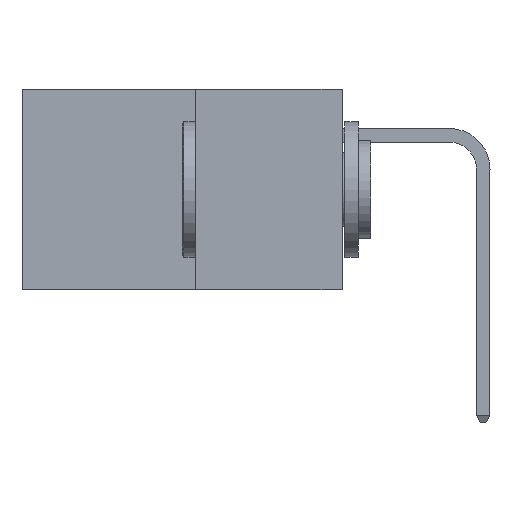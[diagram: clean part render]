
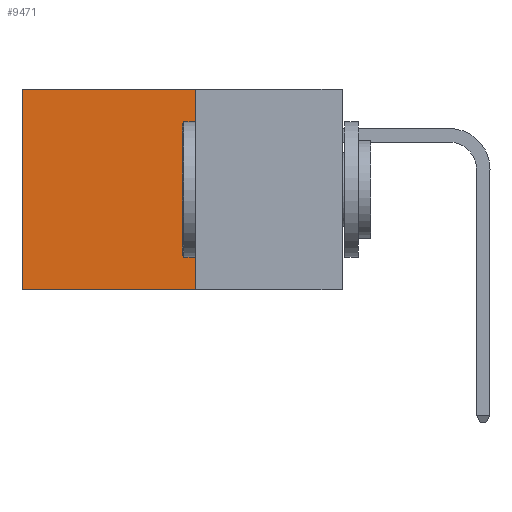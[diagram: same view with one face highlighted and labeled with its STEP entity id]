
A CAD part, left-side view. The second image highlights one B-rep face of the part: STEP entity #9471.
In plain terms, the highlighted planar face has unit normal (-1, 0, 0).
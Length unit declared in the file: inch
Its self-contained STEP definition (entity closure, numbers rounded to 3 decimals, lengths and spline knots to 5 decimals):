
#259 = VECTOR ( 'NONE', #9777, 39.37008 ) ;
#512 = CARTESIAN_POINT ( 'NONE',  ( 0.277, 0.59, -0.37 ) ) ;
#874 = PLANE ( 'NONE',  #8660 ) ;
#1087 = EDGE_CURVE ( 'NONE', #30436, #26529, #21596, .T. ) ;
#2315 = CARTESIAN_POINT ( 'NONE',  ( 0.277, 0.27, 0. ) ) ;
#2369 = CARTESIAN_POINT ( 'NONE',  ( 0.277, 0.27, -0.37 ) ) ;
#3928 = CARTESIAN_POINT ( 'NONE',  ( 0.277, 0.27, -0.37 ) ) ;
#5010 = ORIENTED_EDGE ( 'NONE', *, *, #18793, .F. ) ;
#5689 = VECTOR ( 'NONE', #22698, 39.37008 ) ;
#6069 = DIRECTION ( 'NONE',  ( 0., 0., -1. ) ) ;
#7139 = LINE ( 'NONE', #12357, #259 ) ;
#7997 = VECTOR ( 'NONE', #11887, 39.37008 ) ;
#8660 = AXIS2_PLACEMENT_3D ( 'NONE', #18874, #21423, #6069 ) ;
#9471 = ADVANCED_FACE ( 'NONE', ( #9560 ), #874, .F. ) ;
#9560 = FACE_OUTER_BOUND ( 'NONE', #23953, .T. ) ;
#9777 = DIRECTION ( 'NONE',  ( 0., 0., -1. ) ) ;
#9941 = ORIENTED_EDGE ( 'NONE', *, *, #1087, .F. ) ;
#11887 = DIRECTION ( 'NONE',  ( 0., 0., -1. ) ) ;
#12357 = CARTESIAN_POINT ( 'NONE',  ( 0.277, 0.59, -0.37 ) ) ;
#14771 = CARTESIAN_POINT ( 'NONE',  ( 0.277, 0.27, 0. ) ) ;
#18793 = EDGE_CURVE ( 'NONE', #26529, #22008, #29172, .T. ) ;
#18874 = CARTESIAN_POINT ( 'NONE',  ( 0.277, 0.27, -0.37 ) ) ;
#19292 = DIRECTION ( 'NONE',  ( 0., 1., 0. ) ) ;
#20224 = CARTESIAN_POINT ( 'NONE',  ( 0.277, 0.27, -0.37 ) ) ;
#21423 = DIRECTION ( 'NONE',  ( 1., 0., 0. ) ) ;
#21596 = LINE ( 'NONE', #2369, #7997 ) ;
#21741 = EDGE_CURVE ( 'NONE', #23663, #22008, #7139, .T. ) ;
#22008 = VERTEX_POINT ( 'NONE', #512 ) ;
#22698 = DIRECTION ( 'NONE',  ( 0., 1., 0. ) ) ;
#23663 = VERTEX_POINT ( 'NONE', #32714 ) ;
#23953 = EDGE_LOOP ( 'NONE', ( #30876, #5010, #9941, #25243 ) ) ;
#24448 = LINE ( 'NONE', #2315, #5689 ) ;
#25243 = ORIENTED_EDGE ( 'NONE', *, *, #28984, .T. ) ;
#26529 = VERTEX_POINT ( 'NONE', #20224 ) ;
#28388 = VECTOR ( 'NONE', #19292, 39.37008 ) ;
#28984 = EDGE_CURVE ( 'NONE', #30436, #23663, #24448, .T. ) ;
#29172 = LINE ( 'NONE', #3928, #28388 ) ;
#30436 = VERTEX_POINT ( 'NONE', #14771 ) ;
#30876 = ORIENTED_EDGE ( 'NONE', *, *, #21741, .T. ) ;
#32714 = CARTESIAN_POINT ( 'NONE',  ( 0.277, 0.59, 0. ) ) ;
